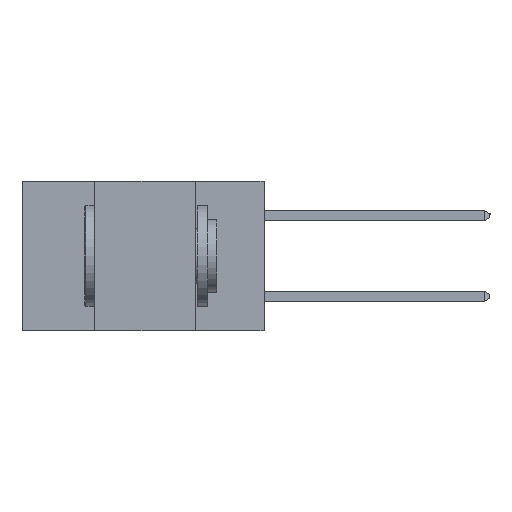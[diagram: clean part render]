
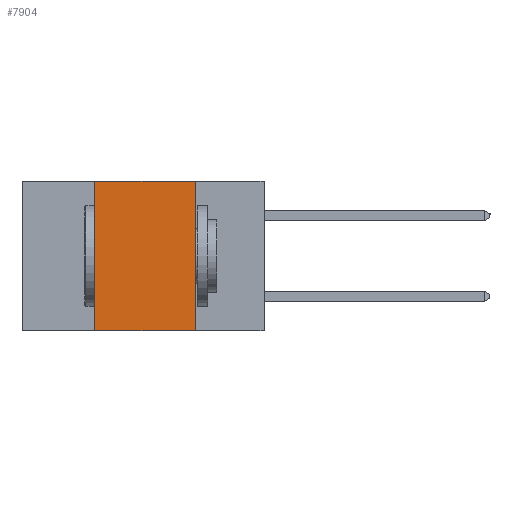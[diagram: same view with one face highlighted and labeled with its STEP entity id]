
A CAD part, left-side view. The second image highlights one B-rep face of the part: STEP entity #7904.
In plain terms, the highlighted planar face has unit normal (-1, 0, 0).
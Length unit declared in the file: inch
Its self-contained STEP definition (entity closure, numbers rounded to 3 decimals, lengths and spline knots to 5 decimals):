
#1071 = VERTEX_POINT ( 'NONE', #4854 ) ;
#1884 = DIRECTION ( 'NONE',  ( 0., -1., 0. ) ) ;
#2060 = ORIENTED_EDGE ( 'NONE', *, *, #18893, .F. ) ;
#2931 = ORIENTED_EDGE ( 'NONE', *, *, #15203, .F. ) ;
#3077 = CARTESIAN_POINT ( 'NONE',  ( 0., 0.42, -0.37 ) ) ;
#3973 = VECTOR ( 'NONE', #19876, 39.37008 ) ;
#4718 = ORIENTED_EDGE ( 'NONE', *, *, #12326, .T. ) ;
#4799 = PLANE ( 'NONE',  #12373 ) ;
#4854 = CARTESIAN_POINT ( 'NONE',  ( 0., 0.42, 0. ) ) ;
#5133 = LINE ( 'NONE', #17376, #6688 ) ;
#6349 = VERTEX_POINT ( 'NONE', #15698 ) ;
#6688 = VECTOR ( 'NONE', #1884, 39.37008 ) ;
#7840 = DIRECTION ( 'NONE',  ( 0., 0., -1. ) ) ;
#7904 = ADVANCED_FACE ( 'NONE', ( #21562 ), #4799, .F. ) ;
#9527 = ORIENTED_EDGE ( 'NONE', *, *, #21535, .F. ) ;
#9658 = LINE ( 'NONE', #21687, #3973 ) ;
#9723 = LINE ( 'NONE', #3077, #15342 ) ;
#10733 = CARTESIAN_POINT ( 'NONE',  ( 0., 0.6, -0.37 ) ) ;
#11516 = DIRECTION ( 'NONE',  ( 0., 0., 1. ) ) ;
#12312 = LINE ( 'NONE', #10733, #19354 ) ;
#12326 = EDGE_CURVE ( 'NONE', #6349, #15113, #12312, .T. ) ;
#12373 = AXIS2_PLACEMENT_3D ( 'NONE', #15014, #21887, #7840 ) ;
#14250 = CARTESIAN_POINT ( 'NONE',  ( 0., 0.17, -0.37 ) ) ;
#14325 = CARTESIAN_POINT ( 'NONE',  ( 0., 0.17, 0. ) ) ;
#15014 = CARTESIAN_POINT ( 'NONE',  ( 0., 0.6, 0. ) ) ;
#15113 = VERTEX_POINT ( 'NONE', #14250 ) ;
#15203 = EDGE_CURVE ( 'NONE', #18676, #15113, #9658, .T. ) ;
#15342 = VECTOR ( 'NONE', #11516, 39.37008 ) ;
#15698 = CARTESIAN_POINT ( 'NONE',  ( 0., 0.42, -0.37 ) ) ;
#16005 = DIRECTION ( 'NONE',  ( 0., -1., 0. ) ) ;
#17376 = CARTESIAN_POINT ( 'NONE',  ( 0., 0.6, 0. ) ) ;
#18057 = EDGE_LOOP ( 'NONE', ( #2931, #9527, #2060, #4718 ) ) ;
#18676 = VERTEX_POINT ( 'NONE', #14325 ) ;
#18893 = EDGE_CURVE ( 'NONE', #6349, #1071, #9723, .T. ) ;
#19354 = VECTOR ( 'NONE', #16005, 39.37008 ) ;
#19876 = DIRECTION ( 'NONE',  ( 0., 0., -1. ) ) ;
#21535 = EDGE_CURVE ( 'NONE', #1071, #18676, #5133, .T. ) ;
#21562 = FACE_OUTER_BOUND ( 'NONE', #18057, .T. ) ;
#21687 = CARTESIAN_POINT ( 'NONE',  ( 0., 0.17, -0.37 ) ) ;
#21887 = DIRECTION ( 'NONE',  ( 1., 0., 0. ) ) ;
